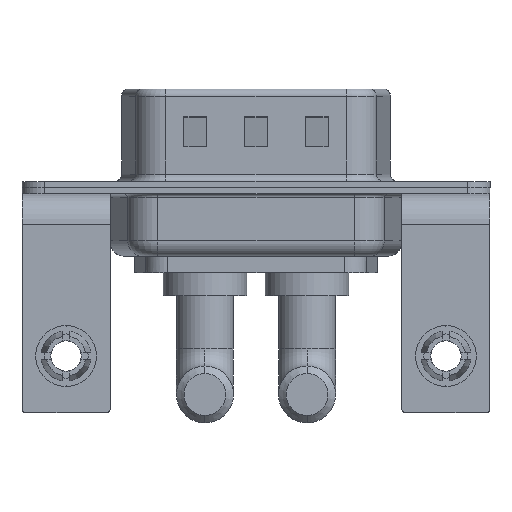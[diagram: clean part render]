
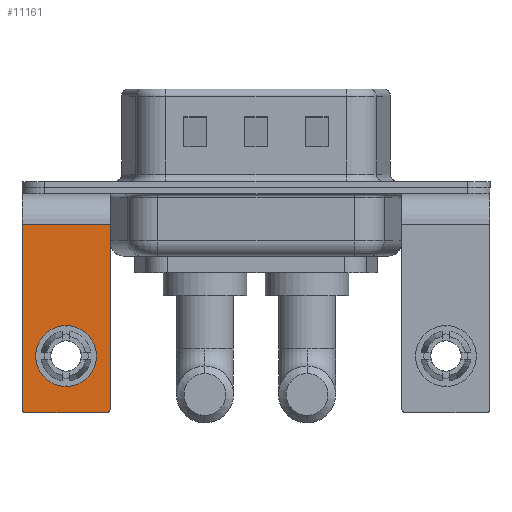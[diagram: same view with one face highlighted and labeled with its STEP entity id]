
A CAD part, front view. The second image highlights one B-rep face of the part: STEP entity #11161.
In plain terms, the highlighted planar face has unit normal (0, -1, 0).
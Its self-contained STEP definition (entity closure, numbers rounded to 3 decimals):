
#40 = DIRECTION ( 'NONE',  ( 0., -1., 0. ) ) ;
#93 = EDGE_CURVE ( 'NONE', #13323, #7953, #10092, .T. ) ;
#137 = EDGE_LOOP ( 'NONE', ( #12833, #518, #10049, #10197, #8628, #1085 ) ) ;
#518 = ORIENTED_EDGE ( 'NONE', *, *, #4802, .T. ) ;
#623 = CIRCLE ( 'NONE', #10217, 2. ) ;
#975 = VERTEX_POINT ( 'NONE', #13462 ) ;
#1085 = ORIENTED_EDGE ( 'NONE', *, *, #2317, .T. ) ;
#1679 = CARTESIAN_POINT ( 'NONE',  ( -2.9, -6.25, -2.4 ) ) ;
#1826 = AXIS2_PLACEMENT_3D ( 'NONE', #4165, #40, #13400 ) ;
#2317 = EDGE_CURVE ( 'NONE', #16687, #11250, #6060, .T. ) ;
#2435 = DIRECTION ( 'NONE',  ( 0., 1., 0. ) ) ;
#2728 = ORIENTED_EDGE ( 'NONE', *, *, #4155, .T. ) ;
#3671 = DIRECTION ( 'NONE',  ( -1., 0., 0. ) ) ;
#3805 = DIRECTION ( 'NONE',  ( 0., 0., -1. ) ) ;
#3917 = VECTOR ( 'NONE', #3805, 1000. ) ;
#3960 = EDGE_CURVE ( 'NONE', #11250, #7470, #14561, .T. ) ;
#4058 = CARTESIAN_POINT ( 'NONE',  ( -2.65, -6.25, -14.8 ) ) ;
#4155 = EDGE_CURVE ( 'NONE', #975, #10983, #623, .T. ) ;
#4165 = CARTESIAN_POINT ( 'NONE',  ( -2.65, -6.25, -14.55 ) ) ;
#4507 = DIRECTION ( 'NONE',  ( 0., -1., 0. ) ) ;
#4802 = EDGE_CURVE ( 'NONE', #7470, #7953, #7571, .T. ) ;
#5209 = CARTESIAN_POINT ( 'NONE',  ( 2.9, -6.25, -14.55 ) ) ;
#5472 = LINE ( 'NONE', #12140, #5945 ) ;
#5610 = FACE_OUTER_BOUND ( 'NONE', #137, .T. ) ;
#5787 = EDGE_LOOP ( 'NONE', ( #11942, #2728 ) ) ;
#5945 = VECTOR ( 'NONE', #10683, 1000. ) ;
#6060 = LINE ( 'NONE', #11536, #15765 ) ;
#6511 = CIRCLE ( 'NONE', #16076, 2. ) ;
#7217 = EDGE_CURVE ( 'NONE', #13323, #12344, #14725, .T. ) ;
#7241 = DIRECTION ( 'NONE',  ( -1., 0., 0. ) ) ;
#7470 = VERTEX_POINT ( 'NONE', #12958 ) ;
#7571 = CIRCLE ( 'NONE', #1826, 0.25 ) ;
#7766 = CARTESIAN_POINT ( 'NONE',  ( 0., -6.25, -11.07 ) ) ;
#7953 = VERTEX_POINT ( 'NONE', #4058 ) ;
#8401 = VECTOR ( 'NONE', #3671, 1000. ) ;
#8628 = ORIENTED_EDGE ( 'NONE', *, *, #14490, .F. ) ;
#9719 = DIRECTION ( 'NONE',  ( 0., 0., 1. ) ) ;
#10049 = ORIENTED_EDGE ( 'NONE', *, *, #93, .F. ) ;
#10092 = LINE ( 'NONE', #12478, #8401 ) ;
#10159 = DIRECTION ( 'NONE',  ( 0., 0., 1. ) ) ;
#10197 = ORIENTED_EDGE ( 'NONE', *, *, #7217, .T. ) ;
#10217 = AXIS2_PLACEMENT_3D ( 'NONE', #7766, #13962, #10266 ) ;
#10266 = DIRECTION ( 'NONE',  ( 0., 0., 1. ) ) ;
#10300 = CARTESIAN_POINT ( 'NONE',  ( -2.9, -6.25, -2.4 ) ) ;
#10371 = AXIS2_PLACEMENT_3D ( 'NONE', #16228, #4507, #9719 ) ;
#10683 = DIRECTION ( 'NONE',  ( 0., 0., -1. ) ) ;
#10983 = VERTEX_POINT ( 'NONE', #15387 ) ;
#11083 = AXIS2_PLACEMENT_3D ( 'NONE', #12203, #14588, #13407 ) ;
#11130 = CARTESIAN_POINT ( 'NONE',  ( 2.65, -6.25, -14.8 ) ) ;
#11161 = ADVANCED_FACE ( 'NONE', ( #12054, #5610 ), #14516, .F. ) ;
#11250 = VERTEX_POINT ( 'NONE', #1679 ) ;
#11536 = CARTESIAN_POINT ( 'NONE',  ( 2.9, -6.25, -2.4 ) ) ;
#11942 = ORIENTED_EDGE ( 'NONE', *, *, #15136, .T. ) ;
#12054 = FACE_BOUND ( 'NONE', #5787, .T. ) ;
#12140 = CARTESIAN_POINT ( 'NONE',  ( 2.9, -6.25, -2.4 ) ) ;
#12203 = CARTESIAN_POINT ( 'NONE',  ( 2.9, -6.25, -2.4 ) ) ;
#12344 = VERTEX_POINT ( 'NONE', #5209 ) ;
#12478 = CARTESIAN_POINT ( 'NONE',  ( 2.9, -6.25, -14.8 ) ) ;
#12833 = ORIENTED_EDGE ( 'NONE', *, *, #3960, .T. ) ;
#12958 = CARTESIAN_POINT ( 'NONE',  ( -2.9, -6.25, -14.55 ) ) ;
#13323 = VERTEX_POINT ( 'NONE', #11130 ) ;
#13400 = DIRECTION ( 'NONE',  ( 0., 0., 1. ) ) ;
#13407 = DIRECTION ( 'NONE',  ( 0., 0., 1. ) ) ;
#13462 = CARTESIAN_POINT ( 'NONE',  ( 0., -6.25, -9.07 ) ) ;
#13962 = DIRECTION ( 'NONE',  ( 0., 1., 0. ) ) ;
#14156 = CARTESIAN_POINT ( 'NONE',  ( 0., -6.25, -11.07 ) ) ;
#14490 = EDGE_CURVE ( 'NONE', #16687, #12344, #5472, .T. ) ;
#14516 = PLANE ( 'NONE',  #11083 ) ;
#14545 = CARTESIAN_POINT ( 'NONE',  ( 2.9, -6.25, -2.4 ) ) ;
#14561 = LINE ( 'NONE', #10300, #3917 ) ;
#14588 = DIRECTION ( 'NONE',  ( 0., 1., 0. ) ) ;
#14725 = CIRCLE ( 'NONE', #10371, 0.25 ) ;
#15136 = EDGE_CURVE ( 'NONE', #10983, #975, #6511, .T. ) ;
#15387 = CARTESIAN_POINT ( 'NONE',  ( 0., -6.25, -13.07 ) ) ;
#15765 = VECTOR ( 'NONE', #7241, 1000. ) ;
#16076 = AXIS2_PLACEMENT_3D ( 'NONE', #14156, #2435, #10159 ) ;
#16228 = CARTESIAN_POINT ( 'NONE',  ( 2.65, -6.25, -14.55 ) ) ;
#16687 = VERTEX_POINT ( 'NONE', #14545 ) ;
